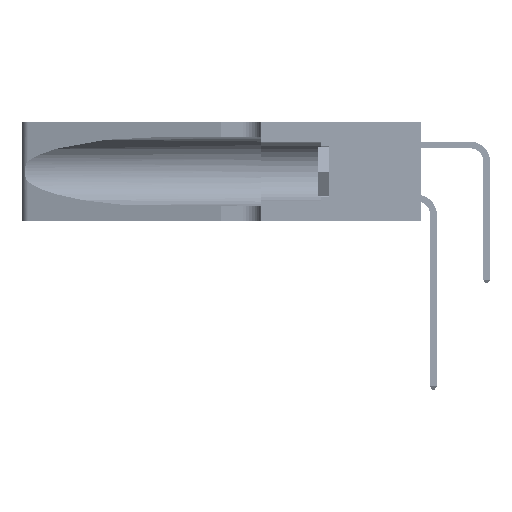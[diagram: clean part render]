
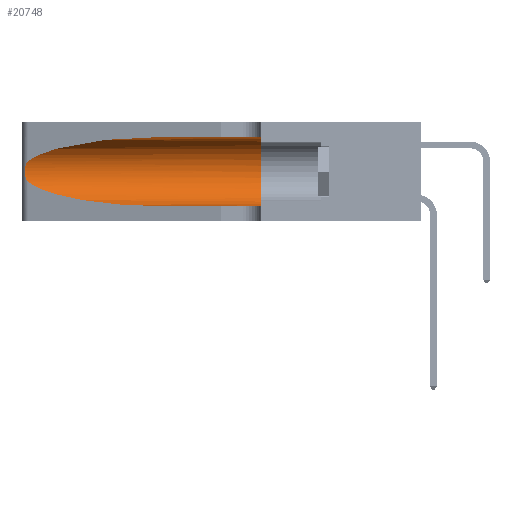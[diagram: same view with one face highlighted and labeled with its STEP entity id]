
A CAD part, left-side view. The second image highlights one B-rep face of the part: STEP entity #20748.
In plain terms, the highlighted cylindrical face has radius 3.308 mm (diameter 6.617 mm), a partial arc.
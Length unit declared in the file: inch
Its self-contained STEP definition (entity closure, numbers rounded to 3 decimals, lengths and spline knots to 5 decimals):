
#194 = VERTEX_POINT ( 'NONE', #34864 ) ;
#1357 = VERTEX_POINT ( 'NONE', #16176 ) ;
#1524 = ORIENTED_EDGE ( 'NONE', *, *, #22145, .T. ) ;
#1945 = AXIS2_PLACEMENT_3D ( 'NONE', #32095, #10258, #35731 ) ;
#2135 = VECTOR ( 'NONE', #37553, 39.37008 ) ;
#2301 = EDGE_CURVE ( 'NONE', #36339, #194, #8331, .T. ) ;
#2490 = CARTESIAN_POINT ( 'NONE',  ( 0.25639, 1.23186, 0.15144 ) ) ;
#4688 = EDGE_LOOP ( 'NONE', ( #34815, #22243, #1524, #34710, #11170, #9438 ) ) ;
#5719 = DIRECTION ( 'NONE',  ( 0., 0., -1. ) ) ;
#5976 = EDGE_CURVE ( 'NONE', #1357, #39375, #45613, .T. ) ;
#6051 = CARTESIAN_POINT ( 'NONE',  ( 0.25487, 1.22718, 0.22369 ) ) ;
#6217 = CARTESIAN_POINT ( 'NONE',  ( 0.25487, 1.22718, 0.14631 ) ) ;
#8331 = CIRCLE ( 'NONE', #1945, 0.13025 ) ;
#9438 = ORIENTED_EDGE ( 'NONE', *, *, #19105, .F. ) ;
#9767 = CARTESIAN_POINT ( 'NONE',  ( 0.25639, 1.23184, 0.21858 ) ) ;
#10077 = VECTOR ( 'NONE', #38215, 39.37008 ) ;
#10258 = DIRECTION ( 'NONE',  ( 0., 1., 0. ) ) ;
#11170 = ORIENTED_EDGE ( 'NONE', *, *, #2301, .F. ) ;
#12461 = CYLINDRICAL_SURFACE ( 'NONE', #13982, 0.13025 ) ;
#13049 = CARTESIAN_POINT ( 'NONE',  ( 0.1305, 0.72297, 0.31525 ) ) ;
#13333 =( BOUNDED_CURVE ( )  B_SPLINE_CURVE ( 3, ( #13049, #16560, #45724, #24063 ),
 .UNSPECIFIED., .F., .F. ) 
 B_SPLINE_CURVE_WITH_KNOTS ( ( 4, 4 ),
 ( 1.5708, 2.84003 ),
 .UNSPECIFIED. ) 
 CURVE ( )  GEOMETRIC_REPRESENTATION_ITEM ( )  RATIONAL_B_SPLINE_CURVE ( ( 1., 0.87, 0.87, 1. ) ) 
 REPRESENTATION_ITEM ( '' )  );
#13441 = CARTESIAN_POINT ( 'NONE',  ( 0.25854, 1.2359, 0.20912 ) ) ;
#13810 = CARTESIAN_POINT ( 'NONE',  ( 0.2373, 1.15595, 0.08982 ) ) ;
#13982 = AXIS2_PLACEMENT_3D ( 'NONE', #27619, #27473, #5719 ) ;
#15324 = CARTESIAN_POINT ( 'NONE',  ( 0.25487, 1.22718, 0.14631 ) ) ;
#16176 = CARTESIAN_POINT ( 'NONE',  ( 0.25487, 1.22718, 0.22369 ) ) ;
#16560 = CARTESIAN_POINT ( 'NONE',  ( 0.18966, 0.96281, 0.31525 ) ) ;
#17117 = CARTESIAN_POINT ( 'NONE',  ( 0.26075, 1.23896, 0.19203 ) ) ;
#18022 = CARTESIAN_POINT ( 'NONE',  ( 0.1305, 0.72297, 0.31525 ) ) ;
#19105 = EDGE_CURVE ( 'NONE', #25542, #36339, #29471, .T. ) ;
#20748 = ADVANCED_FACE ( 'NONE', ( #41446 ), #12461, .F. ) ;
#20796 = CARTESIAN_POINT ( 'NONE',  ( 0.26017, 1.23833, 0.17102 ) ) ;
#21171 = CARTESIAN_POINT ( 'NONE',  ( 0.1305, 0.72297, 0.05475 ) ) ;
#22145 = EDGE_CURVE ( 'NONE', #39375, #29734, #25329, .T. ) ;
#22243 = ORIENTED_EDGE ( 'NONE', *, *, #5976, .T. ) ;
#23117 = CARTESIAN_POINT ( 'NONE',  ( 0.1305, 1.61858, 0.05475 ) ) ;
#24063 = CARTESIAN_POINT ( 'NONE',  ( 0.25487, 1.22718, 0.22369 ) ) ;
#24455 = CARTESIAN_POINT ( 'NONE',  ( 0.25789, 1.23486, 0.15765 ) ) ;
#25329 =( BOUNDED_CURVE ( )  B_SPLINE_CURVE ( 3, ( #46304, #13810, #42855, #21171 ),
 .UNSPECIFIED., .F., .F. ) 
 B_SPLINE_CURVE_WITH_KNOTS ( ( 4, 4 ),
 ( 3.44316, 4.71239 ),
 .UNSPECIFIED. ) 
 CURVE ( )  GEOMETRIC_REPRESENTATION_ITEM ( )  RATIONAL_B_SPLINE_CURVE ( ( 1., 0.87, 0.87, 1. ) ) 
 REPRESENTATION_ITEM ( '' )  );
#25542 = VERTEX_POINT ( 'NONE', #18022 ) ;
#26922 = EDGE_CURVE ( 'NONE', #29734, #194, #31315, .T. ) ;
#27473 = DIRECTION ( 'NONE',  ( 0., -1., 0. ) ) ;
#27619 = CARTESIAN_POINT ( 'NONE',  ( 0.1305, 1.61858, 0.185 ) ) ;
#28100 = CARTESIAN_POINT ( 'NONE',  ( 0.25555, 1.22993, 0.14849 ) ) ;
#29471 = LINE ( 'NONE', #34575, #10077 ) ;
#29734 = VERTEX_POINT ( 'NONE', #38581 ) ;
#31315 = LINE ( 'NONE', #23117, #2135 ) ;
#31588 = CARTESIAN_POINT ( 'NONE',  ( 0.25555, 1.22994, 0.2215 ) ) ;
#32095 = CARTESIAN_POINT ( 'NONE',  ( 0.1305, 0.35, 0.185 ) ) ;
#32539 = CARTESIAN_POINT ( 'NONE',  ( 0.1305, 0.35, 0.31525 ) ) ;
#34575 = CARTESIAN_POINT ( 'NONE',  ( 0.1305, 1.61858, 0.31525 ) ) ;
#34710 = ORIENTED_EDGE ( 'NONE', *, *, #26922, .T. ) ;
#34815 = ORIENTED_EDGE ( 'NONE', *, *, #41665, .T. ) ;
#34864 = CARTESIAN_POINT ( 'NONE',  ( 0.1305, 0.35, 0.05475 ) ) ;
#35232 = CARTESIAN_POINT ( 'NONE',  ( 0.25787, 1.23484, 0.2124 ) ) ;
#35731 = DIRECTION ( 'NONE',  ( 0., 0., 1. ) ) ;
#36339 = VERTEX_POINT ( 'NONE', #32539 ) ;
#37553 = DIRECTION ( 'NONE',  ( 0., -1., 0. ) ) ;
#38215 = DIRECTION ( 'NONE',  ( 0., -1., 0. ) ) ;
#38581 = CARTESIAN_POINT ( 'NONE',  ( 0.1305, 0.72297, 0.05475 ) ) ;
#38868 = CARTESIAN_POINT ( 'NONE',  ( 0.26018, 1.23835, 0.19895 ) ) ;
#39375 = VERTEX_POINT ( 'NONE', #15324 ) ;
#41446 = FACE_OUTER_BOUND ( 'NONE', #4688, .T. ) ;
#41665 = EDGE_CURVE ( 'NONE', #25542, #1357, #13333, .T. ) ;
#42496 = CARTESIAN_POINT ( 'NONE',  ( 0.26075, 1.23896, 0.178 ) ) ;
#42855 = CARTESIAN_POINT ( 'NONE',  ( 0.18966, 0.96281, 0.05475 ) ) ;
#45613 = B_SPLINE_CURVE_WITH_KNOTS ( 'NONE', 3,
 ( #6051, #31588, #9767, #35232, #13441, #38868, #17117, #42496, #20796, #46098, #24455, #2490, #28100, #6217 ),
 .UNSPECIFIED., .F., .F.,
 ( 4, 2, 2, 2, 2, 2, 4 ),
 ( 0., 0.00027, 0.00053, 0.00107, 0.0016, 0.00187, 0.00214 ),
 .UNSPECIFIED. ) ;
#45724 = CARTESIAN_POINT ( 'NONE',  ( 0.2373, 1.15595, 0.28018 ) ) ;
#46098 = CARTESIAN_POINT ( 'NONE',  ( 0.25856, 1.23593, 0.16098 ) ) ;
#46304 = CARTESIAN_POINT ( 'NONE',  ( 0.25487, 1.22718, 0.14631 ) ) ;
